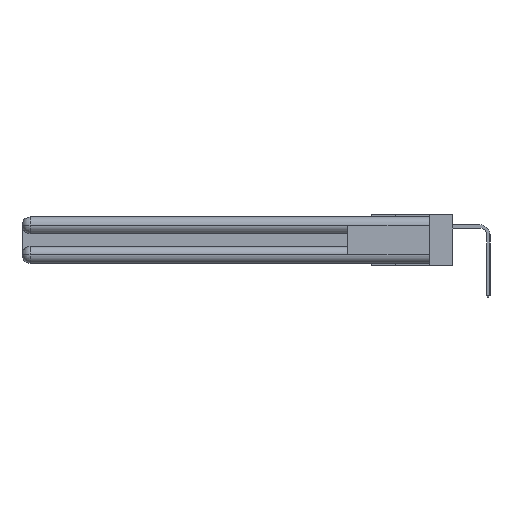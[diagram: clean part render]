
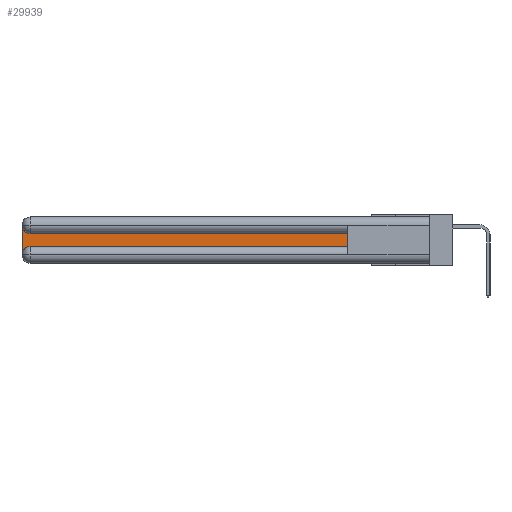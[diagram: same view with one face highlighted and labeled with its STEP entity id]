
A CAD part, left-side view. The second image highlights one B-rep face of the part: STEP entity #29939.
In plain terms, the highlighted planar face has unit normal (-1, 0, 0).
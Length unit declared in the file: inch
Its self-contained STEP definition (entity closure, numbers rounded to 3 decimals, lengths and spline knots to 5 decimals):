
#714 = EDGE_CURVE ( 'NONE', #17947, #5559, #4011, .T. ) ;
#2048 = CARTESIAN_POINT ( 'NONE',  ( 0.075, 0.6, -0.2175 ) ) ;
#2337 = EDGE_CURVE ( 'NONE', #27629, #13133, #18630, .T. ) ;
#2886 = CARTESIAN_POINT ( 'NONE',  ( 0.075, 3., -0.2175 ) ) ;
#3779 = AXIS2_PLACEMENT_3D ( 'NONE', #19275, #28785, #12085 ) ;
#4011 = LINE ( 'NONE', #14550, #10653 ) ;
#4133 = ORIENTED_EDGE ( 'NONE', *, *, #2337, .T. ) ;
#5508 = VECTOR ( 'NONE', #16651, 39.37008 ) ;
#5559 = VERTEX_POINT ( 'NONE', #2048 ) ;
#6676 = CARTESIAN_POINT ( 'NONE',  ( 0.075, 2.94, -0.2775 ) ) ;
#8088 = CARTESIAN_POINT ( 'NONE',  ( 0.075, 2.94, -0.1225 ) ) ;
#8206 = ORIENTED_EDGE ( 'NONE', *, *, #714, .T. ) ;
#9436 = CARTESIAN_POINT ( 'NONE',  ( 0.075, 2.94, -0.0625 ) ) ;
#9805 = EDGE_CURVE ( 'NONE', #17690, #17947, #30022, .T. ) ;
#10180 = LINE ( 'NONE', #2886, #24850 ) ;
#10653 = VECTOR ( 'NONE', #19997, 39.37008 ) ;
#11382 = DIRECTION ( 'NONE',  ( 0., 0., -1. ) ) ;
#11594 = VERTEX_POINT ( 'NONE', #26612 ) ;
#12085 = DIRECTION ( 'NONE',  ( 0., 0., -1. ) ) ;
#12386 = PLANE ( 'NONE',  #3779 ) ;
#13133 = VERTEX_POINT ( 'NONE', #22112 ) ;
#13283 = ORIENTED_EDGE ( 'NONE', *, *, #19059, .T. ) ;
#13423 = EDGE_LOOP ( 'NONE', ( #16242, #4133, #13283, #26388, #8206, #20638 ) ) ;
#14219 = DIRECTION ( 'NONE',  ( 0., 0., -1. ) ) ;
#14550 = CARTESIAN_POINT ( 'NONE',  ( 0.075, 0.6, -0.2175 ) ) ;
#16242 = ORIENTED_EDGE ( 'NONE', *, *, #29316, .T. ) ;
#16651 = DIRECTION ( 'NONE',  ( 0., 1., 0. ) ) ;
#17551 = FACE_OUTER_BOUND ( 'NONE', #13423, .T. ) ;
#17685 = DIRECTION ( 'NONE',  ( 0., 0., 1. ) ) ;
#17690 = VERTEX_POINT ( 'NONE', #29341 ) ;
#17760 = EDGE_CURVE ( 'NONE', #5559, #11594, #25289, .T. ) ;
#17947 = VERTEX_POINT ( 'NONE', #21077 ) ;
#18630 = CIRCLE ( 'NONE', #29270, 0.06 ) ;
#19059 = EDGE_CURVE ( 'NONE', #13133, #17690, #10180, .T. ) ;
#19275 = CARTESIAN_POINT ( 'NONE',  ( 0.075, 3., -0.1225 ) ) ;
#19997 = DIRECTION ( 'NONE',  ( 0., -1., 0. ) ) ;
#20638 = ORIENTED_EDGE ( 'NONE', *, *, #17760, .T. ) ;
#21077 = CARTESIAN_POINT ( 'NONE',  ( 0.075, 2.94, -0.2175 ) ) ;
#21358 = DIRECTION ( 'NONE',  ( 0., 0., -1. ) ) ;
#22112 = CARTESIAN_POINT ( 'NONE',  ( 0.075, 3., -0.0625 ) ) ;
#23109 = DIRECTION ( 'NONE',  ( 1., 0., 0. ) ) ;
#23749 = CARTESIAN_POINT ( 'NONE',  ( 0.075, 0.6, -0.1225 ) ) ;
#24581 = LINE ( 'NONE', #23749, #5508 ) ;
#24850 = VECTOR ( 'NONE', #21358, 39.37008 ) ;
#25289 = LINE ( 'NONE', #29758, #27485 ) ;
#25916 = DIRECTION ( 'NONE',  ( 1., 0., 0. ) ) ;
#26388 = ORIENTED_EDGE ( 'NONE', *, *, #9805, .T. ) ;
#26612 = CARTESIAN_POINT ( 'NONE',  ( 0.075, 0.6, -0.1225 ) ) ;
#26802 = AXIS2_PLACEMENT_3D ( 'NONE', #6676, #23109, #11382 ) ;
#27485 = VECTOR ( 'NONE', #17685, 39.37008 ) ;
#27629 = VERTEX_POINT ( 'NONE', #8088 ) ;
#28785 = DIRECTION ( 'NONE',  ( 1., 0., 0. ) ) ;
#29270 = AXIS2_PLACEMENT_3D ( 'NONE', #9436, #25916, #14219 ) ;
#29316 = EDGE_CURVE ( 'NONE', #11594, #27629, #24581, .T. ) ;
#29341 = CARTESIAN_POINT ( 'NONE',  ( 0.075, 3., -0.2775 ) ) ;
#29758 = CARTESIAN_POINT ( 'NONE',  ( 0.075, 0.6, -0.2175 ) ) ;
#29939 = ADVANCED_FACE ( 'NONE', ( #17551 ), #12386, .F. ) ;
#30022 = CIRCLE ( 'NONE', #26802, 0.06 ) ;
